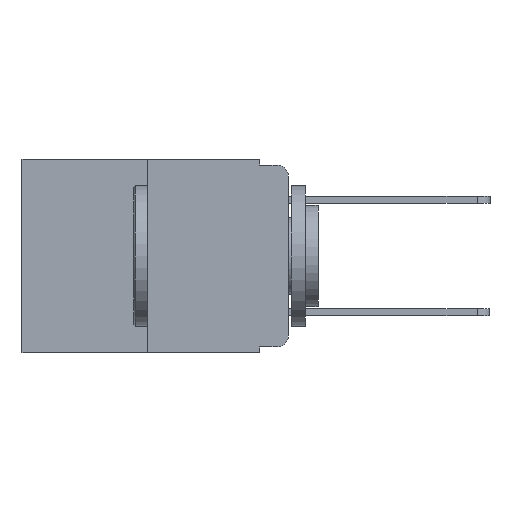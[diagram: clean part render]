
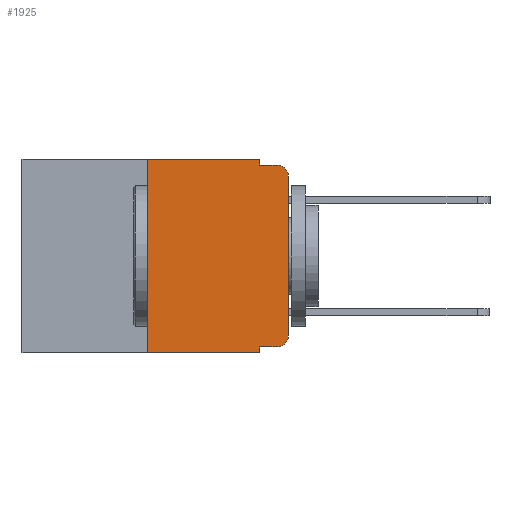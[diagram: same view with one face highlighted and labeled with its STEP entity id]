
A CAD part, left-side view. The second image highlights one B-rep face of the part: STEP entity #1925.
In plain terms, the highlighted planar face has unit normal (-1, 0, 0).
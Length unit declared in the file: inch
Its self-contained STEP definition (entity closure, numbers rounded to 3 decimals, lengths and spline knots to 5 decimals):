
#83 = ORIENTED_EDGE ( 'NONE', *, *, #1582, .T. ) ;
#215 = DIRECTION ( 'NONE',  ( 0., 0., 1. ) ) ;
#242 = CARTESIAN_POINT ( 'NONE',  ( 0., 0.02, -0.03 ) ) ;
#829 = VERTEX_POINT ( 'NONE', #10445 ) ;
#1115 = AXIS2_PLACEMENT_3D ( 'NONE', #5142, #5139, #3093 ) ;
#1166 = ORIENTED_EDGE ( 'NONE', *, *, #6417, .F. ) ;
#1442 = DIRECTION ( 'NONE',  ( 0., 0., -1. ) ) ;
#1495 = VECTOR ( 'NONE', #4592, 39.37008 ) ;
#1535 = EDGE_CURVE ( 'NONE', #2307, #4825, #7871, .T. ) ;
#1552 = EDGE_CURVE ( 'NONE', #2491, #6107, #2431, .T. ) ;
#1582 = EDGE_CURVE ( 'NONE', #6107, #4796, #4733, .T. ) ;
#1656 = EDGE_CURVE ( 'NONE', #6583, #6681, #3000, .T. ) ;
#1680 = EDGE_CURVE ( 'NONE', #829, #4796, #5700, .T. ) ;
#1682 = EDGE_CURVE ( 'NONE', #2307, #2069, #12443, .T. ) ;
#1703 = EDGE_CURVE ( 'NONE', #4825, #2491, #11939, .T. ) ;
#1705 = EDGE_CURVE ( 'NONE', #8615, #829, #7471, .T. ) ;
#1795 = CARTESIAN_POINT ( 'NONE',  ( 0., 0., -0.313 ) ) ;
#1901 = DIRECTION ( 'NONE',  ( -1., 0., 0. ) ) ;
#1908 = ORIENTED_EDGE ( 'NONE', *, *, #7020, .T. ) ;
#1925 = ADVANCED_FACE ( 'NONE', ( #6032 ), #11376, .F. ) ;
#2069 = VERTEX_POINT ( 'NONE', #9059 ) ;
#2072 = VECTOR ( 'NONE', #7231, 39.37008 ) ;
#2222 = ORIENTED_EDGE ( 'NONE', *, *, #1705, .F. ) ;
#2307 = VERTEX_POINT ( 'NONE', #9941 ) ;
#2357 = ORIENTED_EDGE ( 'NONE', *, *, #1703, .T. ) ;
#2431 = LINE ( 'NONE', #7263, #10165 ) ;
#2491 = VERTEX_POINT ( 'NONE', #1795 ) ;
#2597 = ORIENTED_EDGE ( 'NONE', *, *, #1680, .F. ) ;
#2652 = ORIENTED_EDGE ( 'NONE', *, *, #1682, .F. ) ;
#2945 = DIRECTION ( 'NONE',  ( 0., 0., -1. ) ) ;
#3000 = LINE ( 'NONE', #8344, #8273 ) ;
#3093 = DIRECTION ( 'NONE',  ( 0., 0., -1. ) ) ;
#3174 = LINE ( 'NONE', #5526, #5872 ) ;
#3666 = DIRECTION ( 'NONE',  ( 1., 0., 0. ) ) ;
#4441 = LINE ( 'NONE', #6640, #11622 ) ;
#4592 = DIRECTION ( 'NONE',  ( 0., 0., -1. ) ) ;
#4733 = CIRCLE ( 'NONE', #11946, 0.02 ) ;
#4796 = VERTEX_POINT ( 'NONE', #11151 ) ;
#4825 = VERTEX_POINT ( 'NONE', #5940 ) ;
#4952 = CARTESIAN_POINT ( 'NONE',  ( 0., 0.051, 0. ) ) ;
#5006 = CARTESIAN_POINT ( 'NONE',  ( 0., 0.051, -0.01 ) ) ;
#5139 = DIRECTION ( 'NONE',  ( -1., 0., 0. ) ) ;
#5142 = CARTESIAN_POINT ( 'NONE',  ( 0., 0.02, -0.313 ) ) ;
#5336 = VECTOR ( 'NONE', #5522, 39.37008 ) ;
#5337 = CARTESIAN_POINT ( 'NONE',  ( 0., 0.473, 0. ) ) ;
#5522 = DIRECTION ( 'NONE',  ( 0., -1., 0. ) ) ;
#5526 = CARTESIAN_POINT ( 'NONE',  ( 0., 0.473, -0.343 ) ) ;
#5700 = LINE ( 'NONE', #5006, #5336 ) ;
#5872 = VECTOR ( 'NONE', #12576, 39.37008 ) ;
#5924 = CARTESIAN_POINT ( 'NONE',  ( 0., 0.051, 0. ) ) ;
#5940 = CARTESIAN_POINT ( 'NONE',  ( 0., 0.02, -0.333 ) ) ;
#6032 = FACE_OUTER_BOUND ( 'NONE', #8136, .T. ) ;
#6107 = VERTEX_POINT ( 'NONE', #7911 ) ;
#6228 = CARTESIAN_POINT ( 'NONE',  ( 0., 0.051, -0.333 ) ) ;
#6417 = EDGE_CURVE ( 'NONE', #6681, #8615, #4441, .T. ) ;
#6583 = VERTEX_POINT ( 'NONE', #8448 ) ;
#6640 = CARTESIAN_POINT ( 'NONE',  ( 0., 0.473, 0. ) ) ;
#6681 = VERTEX_POINT ( 'NONE', #11960 ) ;
#6929 = ORIENTED_EDGE ( 'NONE', *, *, #1552, .T. ) ;
#7020 = EDGE_CURVE ( 'NONE', #6583, #2069, #3174, .T. ) ;
#7142 = CARTESIAN_POINT ( 'NONE',  ( 0., 0.051, 0. ) ) ;
#7231 = DIRECTION ( 'NONE',  ( 0., -1., 0. ) ) ;
#7263 = CARTESIAN_POINT ( 'NONE',  ( 0., 0., 0. ) ) ;
#7471 = LINE ( 'NONE', #5924, #1495 ) ;
#7517 = ORIENTED_EDGE ( 'NONE', *, *, #1535, .T. ) ;
#7614 = DIRECTION ( 'NONE',  ( 0., -1., 0. ) ) ;
#7871 = LINE ( 'NONE', #6228, #2072 ) ;
#7911 = CARTESIAN_POINT ( 'NONE',  ( 0., 0., -0.03 ) ) ;
#8136 = EDGE_LOOP ( 'NONE', ( #6929, #83, #2597, #2222, #1166, #11626, #1908, #2652, #7517, #2357 ) ) ;
#8273 = VECTOR ( 'NONE', #11250, 39.37008 ) ;
#8344 = CARTESIAN_POINT ( 'NONE',  ( 0., 0.25, 0. ) ) ;
#8448 = CARTESIAN_POINT ( 'NONE',  ( 0., 0.25, -0.343 ) ) ;
#8615 = VERTEX_POINT ( 'NONE', #7142 ) ;
#9059 = CARTESIAN_POINT ( 'NONE',  ( 0., 0.051, -0.343 ) ) ;
#9941 = CARTESIAN_POINT ( 'NONE',  ( 0., 0.051, -0.333 ) ) ;
#10165 = VECTOR ( 'NONE', #215, 39.37008 ) ;
#10445 = CARTESIAN_POINT ( 'NONE',  ( 0., 0.051, -0.01 ) ) ;
#10641 = AXIS2_PLACEMENT_3D ( 'NONE', #5337, #3666, #11381 ) ;
#11151 = CARTESIAN_POINT ( 'NONE',  ( 0., 0.02, -0.01 ) ) ;
#11250 = DIRECTION ( 'NONE',  ( 0., 0., 1. ) ) ;
#11376 = PLANE ( 'NONE',  #10641 ) ;
#11381 = DIRECTION ( 'NONE',  ( 0., 0., -1. ) ) ;
#11622 = VECTOR ( 'NONE', #7614, 39.37008 ) ;
#11626 = ORIENTED_EDGE ( 'NONE', *, *, #1656, .F. ) ;
#11939 = CIRCLE ( 'NONE', #1115, 0.02 ) ;
#11946 = AXIS2_PLACEMENT_3D ( 'NONE', #242, #1901, #1442 ) ;
#11960 = CARTESIAN_POINT ( 'NONE',  ( 0., 0.25, 0. ) ) ;
#12191 = VECTOR ( 'NONE', #2945, 39.37008 ) ;
#12443 = LINE ( 'NONE', #4952, #12191 ) ;
#12576 = DIRECTION ( 'NONE',  ( 0., -1., 0. ) ) ;
